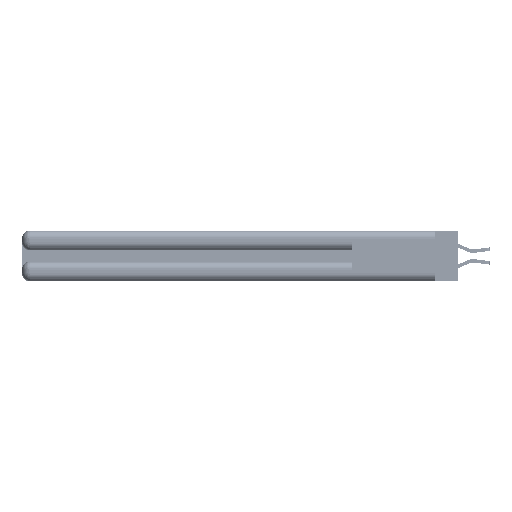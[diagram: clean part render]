
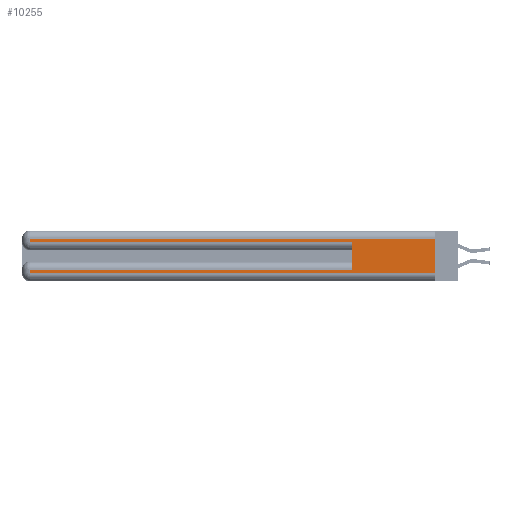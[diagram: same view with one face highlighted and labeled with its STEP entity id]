
A CAD part, left-side view. The second image highlights one B-rep face of the part: STEP entity #10255.
In plain terms, the highlighted planar face has unit normal (-1, 0, 0).
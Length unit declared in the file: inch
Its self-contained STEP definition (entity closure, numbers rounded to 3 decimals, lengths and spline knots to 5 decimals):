
#1195 = DIRECTION ( 'NONE',  ( 0., 0., -1. ) ) ;
#3029 = LINE ( 'NONE', #17310, #4329 ) ;
#3743 = ORIENTED_EDGE ( 'NONE', *, *, #49926, .T. ) ;
#4329 = VECTOR ( 'NONE', #42672, 39.37008 ) ;
#4902 = LINE ( 'NONE', #53097, #14896 ) ;
#4922 = CARTESIAN_POINT ( 'NONE',  ( 0., 0., 0.085 ) ) ;
#6527 = CARTESIAN_POINT ( 'NONE',  ( 0., 2.94, 0.31 ) ) ;
#6573 = PLANE ( 'NONE',  #20621 ) ;
#8564 = CARTESIAN_POINT ( 'NONE',  ( 0., 0.6, 0.145 ) ) ;
#9171 = DIRECTION ( 'NONE',  ( 0., 1., 0. ) ) ;
#9937 = VECTOR ( 'NONE', #10682, 39.37008 ) ;
#10255 = ADVANCED_FACE ( 'NONE', ( #53547 ), #6573, .F. ) ;
#10682 = DIRECTION ( 'NONE',  ( 0., -1., 0. ) ) ;
#12283 = EDGE_CURVE ( 'NONE', #36669, #41286, #47011, .T. ) ;
#14362 = CARTESIAN_POINT ( 'NONE',  ( 0., 2.94, 0.37 ) ) ;
#14896 = VECTOR ( 'NONE', #28156, 39.37008 ) ;
#17079 = LINE ( 'NONE', #25017, #49489 ) ;
#17310 = CARTESIAN_POINT ( 'NONE',  ( 0., 0., 0.285 ) ) ;
#19793 = CARTESIAN_POINT ( 'NONE',  ( 0., 2.94, 0.085 ) ) ;
#20309 = LINE ( 'NONE', #8564, #22973 ) ;
#20621 = AXIS2_PLACEMENT_3D ( 'NONE', #36065, #23295, #31467 ) ;
#22274 = VECTOR ( 'NONE', #1195, 39.37008 ) ;
#22973 = VECTOR ( 'NONE', #45966, 39.37008 ) ;
#23295 = DIRECTION ( 'NONE',  ( 1., 0., 0. ) ) ;
#23783 = ORIENTED_EDGE ( 'NONE', *, *, #39432, .T. ) ;
#25017 = CARTESIAN_POINT ( 'NONE',  ( 0., 2.94, 0.37 ) ) ;
#26180 = VERTEX_POINT ( 'NONE', #34256 ) ;
#26300 = CARTESIAN_POINT ( 'NONE',  ( 0., 0.6, 0.285 ) ) ;
#26456 = VECTOR ( 'NONE', #30815, 39.37008 ) ;
#27392 = ORIENTED_EDGE ( 'NONE', *, *, #38027, .F. ) ;
#28156 = DIRECTION ( 'NONE',  ( 0., 1., 0. ) ) ;
#29080 = DIRECTION ( 'NONE',  ( 0., 0., -1. ) ) ;
#29566 = ORIENTED_EDGE ( 'NONE', *, *, #12283, .T. ) ;
#30141 = VERTEX_POINT ( 'NONE', #46811 ) ;
#30815 = DIRECTION ( 'NONE',  ( 0., 0., -1. ) ) ;
#30991 = ORIENTED_EDGE ( 'NONE', *, *, #46701, .T. ) ;
#31061 = ORIENTED_EDGE ( 'NONE', *, *, #36059, .T. ) ;
#31467 = DIRECTION ( 'NONE',  ( 0., 0., -1. ) ) ;
#32911 = CARTESIAN_POINT ( 'NONE',  ( 0., 2.94, 0.06 ) ) ;
#33725 = CARTESIAN_POINT ( 'NONE',  ( 0., 0., 0.06 ) ) ;
#34256 = CARTESIAN_POINT ( 'NONE',  ( 0., 0., 0.31 ) ) ;
#36059 = EDGE_CURVE ( 'NONE', #48744, #30141, #17079, .T. ) ;
#36065 = CARTESIAN_POINT ( 'NONE',  ( 0., 0., 0.37 ) ) ;
#36669 = VERTEX_POINT ( 'NONE', #32911 ) ;
#37890 = VERTEX_POINT ( 'NONE', #46468 ) ;
#38027 = EDGE_CURVE ( 'NONE', #26180, #41286, #47581, .T. ) ;
#39312 = EDGE_CURVE ( 'NONE', #37890, #49948, #20309, .T. ) ;
#39432 = EDGE_CURVE ( 'NONE', #30141, #49948, #3029, .T. ) ;
#40585 = VECTOR ( 'NONE', #9171, 39.37008 ) ;
#41286 = VERTEX_POINT ( 'NONE', #33725 ) ;
#41516 = EDGE_LOOP ( 'NONE', ( #27392, #47349, #31061, #23783, #52369, #3743, #30991, #29566 ) ) ;
#42672 = DIRECTION ( 'NONE',  ( 0., -1., 0. ) ) ;
#44751 = LINE ( 'NONE', #14362, #22274 ) ;
#44940 = VERTEX_POINT ( 'NONE', #19793 ) ;
#45966 = DIRECTION ( 'NONE',  ( 0., 0., 1. ) ) ;
#46446 = LINE ( 'NONE', #4922, #40585 ) ;
#46468 = CARTESIAN_POINT ( 'NONE',  ( 0., 0.6, 0.085 ) ) ;
#46701 = EDGE_CURVE ( 'NONE', #44940, #36669, #44751, .T. ) ;
#46811 = CARTESIAN_POINT ( 'NONE',  ( 0., 2.94, 0.285 ) ) ;
#47011 = LINE ( 'NONE', #52541, #9937 ) ;
#47349 = ORIENTED_EDGE ( 'NONE', *, *, #48226, .T. ) ;
#47581 = LINE ( 'NONE', #47771, #26456 ) ;
#47771 = CARTESIAN_POINT ( 'NONE',  ( 0., 0., 0.37 ) ) ;
#48226 = EDGE_CURVE ( 'NONE', #26180, #48744, #4902, .T. ) ;
#48744 = VERTEX_POINT ( 'NONE', #6527 ) ;
#49489 = VECTOR ( 'NONE', #29080, 39.37008 ) ;
#49926 = EDGE_CURVE ( 'NONE', #37890, #44940, #46446, .T. ) ;
#49948 = VERTEX_POINT ( 'NONE', #26300 ) ;
#52369 = ORIENTED_EDGE ( 'NONE', *, *, #39312, .F. ) ;
#52541 = CARTESIAN_POINT ( 'NONE',  ( 0., 0., 0.06 ) ) ;
#53097 = CARTESIAN_POINT ( 'NONE',  ( 0., 0., 0.31 ) ) ;
#53547 = FACE_OUTER_BOUND ( 'NONE', #41516, .T. ) ;
